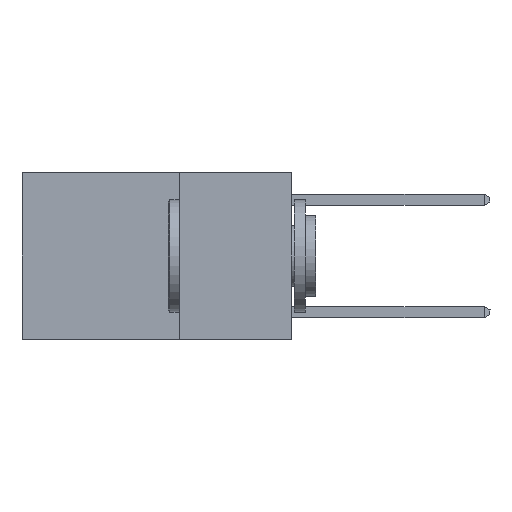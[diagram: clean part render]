
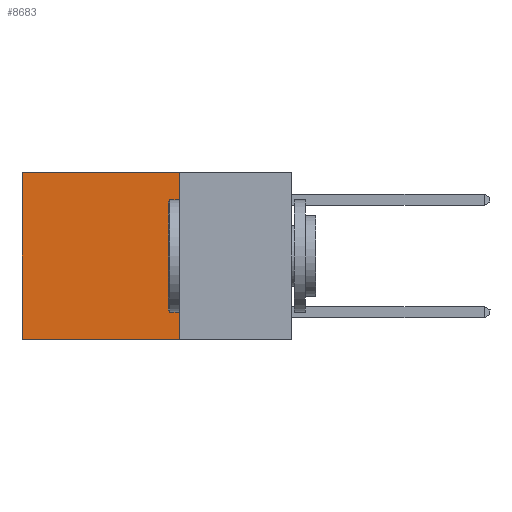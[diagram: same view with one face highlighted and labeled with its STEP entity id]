
A CAD part, left-side view. The second image highlights one B-rep face of the part: STEP entity #8683.
In plain terms, the highlighted planar face has unit normal (-1, 0, 0).
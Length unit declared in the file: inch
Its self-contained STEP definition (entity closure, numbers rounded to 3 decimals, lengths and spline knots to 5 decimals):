
#657 = DIRECTION ( 'NONE',  ( 0., 0., -1. ) ) ;
#2284 = CARTESIAN_POINT ( 'NONE',  ( 0.2625, 0.6, 0. ) ) ;
#2293 = EDGE_CURVE ( 'NONE', #12658, #8075, #15839, .T. ) ;
#3230 = AXIS2_PLACEMENT_3D ( 'NONE', #6069, #7626, #17274 ) ;
#3771 = DIRECTION ( 'NONE',  ( 0., 0., -1. ) ) ;
#3936 = CARTESIAN_POINT ( 'NONE',  ( 0.2625, 0.25, -0.37 ) ) ;
#5437 = VERTEX_POINT ( 'NONE', #6762 ) ;
#6069 = CARTESIAN_POINT ( 'NONE',  ( 0.2625, 0.25, 0. ) ) ;
#6762 = CARTESIAN_POINT ( 'NONE',  ( 0.2625, 0.25, 0. ) ) ;
#6906 = ORIENTED_EDGE ( 'NONE', *, *, #2293, .F. ) ;
#7395 = CARTESIAN_POINT ( 'NONE',  ( 0.2625, 0.6, -0.37 ) ) ;
#7448 = PLANE ( 'NONE',  #3230 ) ;
#7626 = DIRECTION ( 'NONE',  ( 1., 0., 0. ) ) ;
#7644 = CARTESIAN_POINT ( 'NONE',  ( 0.2625, 0.6, 0. ) ) ;
#8014 = ORIENTED_EDGE ( 'NONE', *, *, #17749, .T. ) ;
#8075 = VERTEX_POINT ( 'NONE', #7395 ) ;
#8683 = ADVANCED_FACE ( 'NONE', ( #10480 ), #7448, .F. ) ;
#8739 = DIRECTION ( 'NONE',  ( 0., 1., 0. ) ) ;
#9323 = CARTESIAN_POINT ( 'NONE',  ( 0.2625, 0.25, 0. ) ) ;
#10480 = FACE_OUTER_BOUND ( 'NONE', #15497, .T. ) ;
#11604 = VERTEX_POINT ( 'NONE', #7644 ) ;
#11968 = LINE ( 'NONE', #9323, #14712 ) ;
#12255 = EDGE_CURVE ( 'NONE', #11604, #8075, #14914, .T. ) ;
#12308 = VECTOR ( 'NONE', #16013, 39.37008 ) ;
#12658 = VERTEX_POINT ( 'NONE', #3936 ) ;
#12675 = CARTESIAN_POINT ( 'NONE',  ( 0.2625, 0.25, -0.37 ) ) ;
#12967 = EDGE_CURVE ( 'NONE', #5437, #12658, #11968, .T. ) ;
#13362 = VECTOR ( 'NONE', #8739, 39.37008 ) ;
#13795 = VECTOR ( 'NONE', #3771, 39.37008 ) ;
#14051 = ORIENTED_EDGE ( 'NONE', *, *, #12967, .F. ) ;
#14712 = VECTOR ( 'NONE', #657, 39.37008 ) ;
#14914 = LINE ( 'NONE', #2284, #13795 ) ;
#15497 = EDGE_LOOP ( 'NONE', ( #18002, #6906, #14051, #8014 ) ) ;
#15839 = LINE ( 'NONE', #12675, #13362 ) ;
#16013 = DIRECTION ( 'NONE',  ( 0., 1., 0. ) ) ;
#17274 = DIRECTION ( 'NONE',  ( 0., 0., -1. ) ) ;
#17538 = LINE ( 'NONE', #17627, #12308 ) ;
#17627 = CARTESIAN_POINT ( 'NONE',  ( 0.2625, 0.25, 0. ) ) ;
#17749 = EDGE_CURVE ( 'NONE', #5437, #11604, #17538, .T. ) ;
#18002 = ORIENTED_EDGE ( 'NONE', *, *, #12255, .T. ) ;
